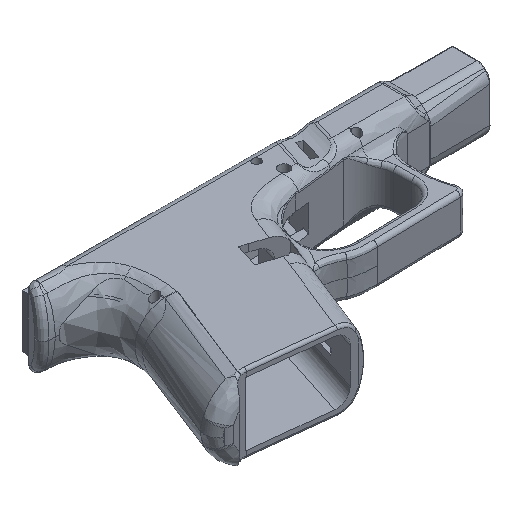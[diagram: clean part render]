
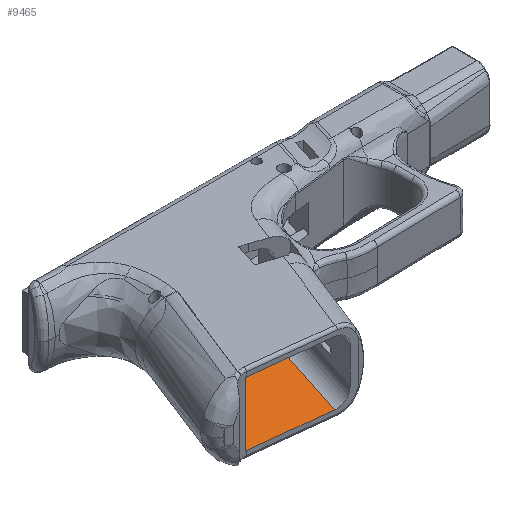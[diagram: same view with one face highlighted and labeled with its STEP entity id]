
A CAD part, isometric view. The second image highlights one B-rep face of the part: STEP entity #9465.
In plain terms, the highlighted planar face has unit normal (0, 0, 1).
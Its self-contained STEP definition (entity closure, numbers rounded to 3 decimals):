
#335=CIRCLE('',#10112,6.);
#1784=FACE_OUTER_BOUND('',#2284,.T.);
#2284=EDGE_LOOP('',(#7376,#7377,#7378,#7379,#7380,#7381,#7382,#7383,#7384,
#7385,#7386,#7387,#7388));
#2659=LINE('',#13259,#3193);
#2815=LINE('',#15936,#3349);
#2882=LINE('',#22722,#3416);
#2913=LINE('',#24416,#3447);
#2914=LINE('',#24418,#3448);
#2915=LINE('',#24420,#3449);
#2916=LINE('',#24421,#3450);
#2917=LINE('',#24423,#3451);
#2918=LINE('',#24425,#3452);
#2919=LINE('',#24426,#3453);
#2920=LINE('',#24428,#3454);
#2921=LINE('',#24429,#3455);
#3193=VECTOR('',#10793,10.);
#3349=VECTOR('',#11185,10.);
#3416=VECTOR('',#11442,10.);
#3447=VECTOR('',#11593,10.);
#3448=VECTOR('',#11594,10.);
#3449=VECTOR('',#11595,10.);
#3450=VECTOR('',#11596,10.);
#3451=VECTOR('',#11597,10.);
#3452=VECTOR('',#11598,10.);
#3453=VECTOR('',#11599,10.);
#3454=VECTOR('',#11600,10.);
#3455=VECTOR('',#11601,1000.);
#3867=VERTEX_POINT('',#13256);
#3868=VERTEX_POINT('',#13258);
#4072=VERTEX_POINT('',#15933);
#4073=VERTEX_POINT('',#15935);
#4279=VERTEX_POINT('',#22719);
#4280=VERTEX_POINT('',#22721);
#4304=VERTEX_POINT('',#23118);
#4358=VERTEX_POINT('',#24415);
#4359=VERTEX_POINT('',#24417);
#4360=VERTEX_POINT('',#24419);
#4361=VERTEX_POINT('',#24422);
#4362=VERTEX_POINT('',#24424);
#4363=VERTEX_POINT('',#24427);
#4864=EDGE_CURVE('',#3867,#3868,#2659,.F.);
#5131=EDGE_CURVE('',#4072,#4073,#2815,.F.);
#5381=EDGE_CURVE('',#4280,#4279,#2882,.T.);
#5413=EDGE_CURVE('',#4304,#4280,#335,.F.);
#5501=EDGE_CURVE('',#4358,#3868,#2913,.T.);
#5502=EDGE_CURVE('',#4359,#3867,#2914,.F.);
#5503=EDGE_CURVE('',#4360,#4359,#2915,.F.);
#5504=EDGE_CURVE('',#4073,#4360,#2916,.F.);
#5505=EDGE_CURVE('',#4361,#4072,#2917,.F.);
#5506=EDGE_CURVE('',#4362,#4361,#2918,.T.);
#5507=EDGE_CURVE('',#4304,#4362,#2919,.T.);
#5508=EDGE_CURVE('',#4363,#4279,#2920,.T.);
#5509=EDGE_CURVE('',#4363,#4358,#2921,.T.);
#7376=ORIENTED_EDGE('',*,*,#5501,.T.);
#7377=ORIENTED_EDGE('',*,*,#4864,.F.);
#7378=ORIENTED_EDGE('',*,*,#5502,.F.);
#7379=ORIENTED_EDGE('',*,*,#5503,.F.);
#7380=ORIENTED_EDGE('',*,*,#5504,.F.);
#7381=ORIENTED_EDGE('',*,*,#5131,.F.);
#7382=ORIENTED_EDGE('',*,*,#5505,.F.);
#7383=ORIENTED_EDGE('',*,*,#5506,.F.);
#7384=ORIENTED_EDGE('',*,*,#5507,.F.);
#7385=ORIENTED_EDGE('',*,*,#5413,.T.);
#7386=ORIENTED_EDGE('',*,*,#5381,.T.);
#7387=ORIENTED_EDGE('',*,*,#5508,.F.);
#7388=ORIENTED_EDGE('',*,*,#5509,.T.);
#9194=PLANE('',#10156);
#9465=ADVANCED_FACE('',(#1784),#9194,.T.);
#10112=AXIS2_PLACEMENT_3D('',#23119,#11479,#11480);
#10156=AXIS2_PLACEMENT_3D('',#24414,#11591,#11592);
#10793=DIRECTION('',(-1.,0.,0.));
#11185=DIRECTION('',(-1.,0.,0.));
#11442=DIRECTION('',(0.994,-0.111,0.));
#11479=DIRECTION('center_axis',(0.,0.,1.));
#11480=DIRECTION('ref_axis',(-0.451,0.893,0.));
#11591=DIRECTION('center_axis',(0.,0.,1.));
#11592=DIRECTION('ref_axis',(1.,0.,0.));
#11593=DIRECTION('',(0.301,0.954,0.));
#11594=DIRECTION('',(0.,-1.,0.));
#11595=DIRECTION('',(-1.,0.,0.));
#11596=DIRECTION('',(0.,1.,0.));
#11597=DIRECTION('',(-0.309,-0.951,0.));
#11598=DIRECTION('',(0.951,-0.309,0.));
#11599=DIRECTION('',(0.309,0.951,0.));
#11600=DIRECTION('',(-0.309,-0.951,0.));
#11601=DIRECTION('',(1.,0.,0.));
#13256=CARTESIAN_POINT('',(62.1,-1.5,-11.75));
#13258=CARTESIAN_POINT('',(69.764,-1.5,-11.75));
#13259=CARTESIAN_POINT('',(61.488,-1.5,-11.75));
#15933=CARTESIAN_POINT('',(47.586,-1.5,-11.75));
#15935=CARTESIAN_POINT('',(52.35,-1.5,-11.75));
#15936=CARTESIAN_POINT('',(61.488,-1.5,-11.75));
#22719=CARTESIAN_POINT('',(41.004,-72.908,-11.75));
#22721=CARTESIAN_POINT('',(11.763,-69.638,-11.75));
#22722=CARTESIAN_POINT('',(12.068,-69.672,-11.75));
#23118=CARTESIAN_POINT('',(11.46,-69.612,-11.75));
#23119=CARTESIAN_POINT('Origin',(11.096,-75.601,-11.75));
#24414=CARTESIAN_POINT('Origin',(-2.2,-1.,-11.75));
#24415=CARTESIAN_POINT('',(65.192,-16.,-11.75));
#24416=CARTESIAN_POINT('',(66.549,-11.698,-11.75));
#24417=CARTESIAN_POINT('',(62.1,-3.,-11.75));
#24418=CARTESIAN_POINT('',(62.1,-53.999,-11.75));
#24419=CARTESIAN_POINT('',(52.35,-3.,-11.75));
#24420=CARTESIAN_POINT('',(46.014,-3.,-11.75));
#24421=CARTESIAN_POINT('',(52.35,-54.999,-11.75));
#24422=CARTESIAN_POINT('',(44.828,-9.989,-11.75));
#24423=CARTESIAN_POINT('',(29.862,-56.051,-11.75));
#24424=CARTESIAN_POINT('',(32.169,-5.875,-11.75));
#24425=CARTESIAN_POINT('',(32.712,-6.052,-11.75));
#24426=CARTESIAN_POINT('',(2.312,-97.765,-11.75));
#24427=CARTESIAN_POINT('',(59.494,-16.,-11.75));
#24428=CARTESIAN_POINT('',(43.969,-63.781,-11.75));
#24429=CARTESIAN_POINT('',(0.,-16.,-11.75));
